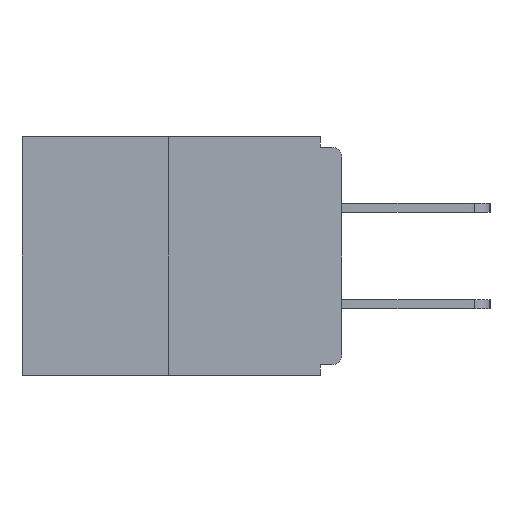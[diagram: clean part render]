
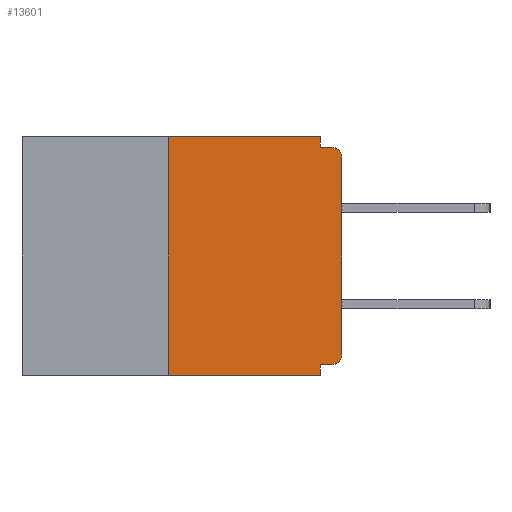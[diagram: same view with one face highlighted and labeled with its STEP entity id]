
A CAD part, left-side view. The second image highlights one B-rep face of the part: STEP entity #13601.
In plain terms, the highlighted planar face has unit normal (-1, 0, 0).
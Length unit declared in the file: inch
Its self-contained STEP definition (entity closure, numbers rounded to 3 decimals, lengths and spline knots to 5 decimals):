
#199 = ORIENTED_EDGE ( 'NONE', *, *, #3254, .F. ) ;
#528 = CARTESIAN_POINT ( 'NONE',  ( 0., 0.015, -0.328 ) ) ;
#533 = VERTEX_POINT ( 'NONE', #11668 ) ;
#868 = LINE ( 'NONE', #8598, #15008 ) ;
#1025 = CARTESIAN_POINT ( 'NONE',  ( 0., 0., 0. ) ) ;
#1148 = DIRECTION ( 'NONE',  ( 0., -1., 0. ) ) ;
#1209 = CARTESIAN_POINT ( 'NONE',  ( 0., 0.25, -0.343 ) ) ;
#1368 = CARTESIAN_POINT ( 'NONE',  ( 0., 0.031, -0.343 ) ) ;
#1601 = LINE ( 'NONE', #5882, #2080 ) ;
#2080 = VECTOR ( 'NONE', #10331, 39.37008 ) ;
#2097 = EDGE_CURVE ( 'NONE', #9857, #6369, #3973, .T. ) ;
#3080 = VERTEX_POINT ( 'NONE', #7480 ) ;
#3254 = EDGE_CURVE ( 'NONE', #533, #16850, #6962, .T. ) ;
#3834 = VECTOR ( 'NONE', #8812, 39.37008 ) ;
#3973 = LINE ( 'NONE', #11247, #7440 ) ;
#4348 = FACE_OUTER_BOUND ( 'NONE', #14300, .T. ) ;
#4618 = VERTEX_POINT ( 'NONE', #8469 ) ;
#5040 = CARTESIAN_POINT ( 'NONE',  ( 0., 0.031, -0.343 ) ) ;
#5282 = EDGE_CURVE ( 'NONE', #18631, #4618, #1601, .T. ) ;
#5661 = EDGE_CURVE ( 'NONE', #16668, #10825, #8485, .T. ) ;
#5882 = CARTESIAN_POINT ( 'NONE',  ( 0., 0.25, 0. ) ) ;
#6029 = PLANE ( 'NONE',  #18758 ) ;
#6369 = VERTEX_POINT ( 'NONE', #8794 ) ;
#6962 = LINE ( 'NONE', #5040, #17421 ) ;
#7039 = ORIENTED_EDGE ( 'NONE', *, *, #16143, .F. ) ;
#7192 = LINE ( 'NONE', #1025, #10149 ) ;
#7356 = ORIENTED_EDGE ( 'NONE', *, *, #10472, .T. ) ;
#7440 = VECTOR ( 'NONE', #1148, 39.37008 ) ;
#7480 = CARTESIAN_POINT ( 'NONE',  ( 0., 0.031, 0. ) ) ;
#7572 = CARTESIAN_POINT ( 'NONE',  ( 0., 0.031, 0. ) ) ;
#7769 = CIRCLE ( 'NONE', #17304, 0.015 ) ;
#8296 = VERTEX_POINT ( 'NONE', #9148 ) ;
#8469 = CARTESIAN_POINT ( 'NONE',  ( 0., 0.25, 0. ) ) ;
#8485 = CIRCLE ( 'NONE', #10786, 0.015 ) ;
#8598 = CARTESIAN_POINT ( 'NONE',  ( 0., 0., -0.328 ) ) ;
#8685 = DIRECTION ( 'NONE',  ( 0., 0., -1. ) ) ;
#8713 = DIRECTION ( 'NONE',  ( 0., 0., -1. ) ) ;
#8794 = CARTESIAN_POINT ( 'NONE',  ( 0., 0.015, -0.015 ) ) ;
#8811 = CARTESIAN_POINT ( 'NONE',  ( 0., 0., -0.313 ) ) ;
#8812 = DIRECTION ( 'NONE',  ( 0., -1., 0. ) ) ;
#9049 = VECTOR ( 'NONE', #15526, 39.37008 ) ;
#9148 = CARTESIAN_POINT ( 'NONE',  ( 0., 0., -0.03 ) ) ;
#9426 = ORIENTED_EDGE ( 'NONE', *, *, #14720, .T. ) ;
#9807 = DIRECTION ( 'NONE',  ( 0., 0., 1. ) ) ;
#9857 = VERTEX_POINT ( 'NONE', #10898 ) ;
#10149 = VECTOR ( 'NONE', #9807, 39.37008 ) ;
#10330 = ORIENTED_EDGE ( 'NONE', *, *, #14773, .F. ) ;
#10331 = DIRECTION ( 'NONE',  ( 0., 0., 1. ) ) ;
#10350 = DIRECTION ( 'NONE',  ( 1., 0., 0. ) ) ;
#10472 = EDGE_CURVE ( 'NONE', #18631, #16850, #12883, .T. ) ;
#10786 = AXIS2_PLACEMENT_3D ( 'NONE', #16102, #13264, #17585 ) ;
#10791 = ORIENTED_EDGE ( 'NONE', *, *, #5282, .F. ) ;
#10825 = VERTEX_POINT ( 'NONE', #8811 ) ;
#10898 = CARTESIAN_POINT ( 'NONE',  ( 0., 0.031, -0.015 ) ) ;
#11247 = CARTESIAN_POINT ( 'NONE',  ( 0., 0., -0.015 ) ) ;
#11385 = LINE ( 'NONE', #17426, #3834 ) ;
#11668 = CARTESIAN_POINT ( 'NONE',  ( 0., 0.031, -0.328 ) ) ;
#11681 = EDGE_CURVE ( 'NONE', #10825, #8296, #7192, .T. ) ;
#11688 = VECTOR ( 'NONE', #16380, 39.37008 ) ;
#12364 = LINE ( 'NONE', #7572, #11688 ) ;
#12883 = LINE ( 'NONE', #18602, #9049 ) ;
#12914 = CARTESIAN_POINT ( 'NONE',  ( 0., 0.015, -0.03 ) ) ;
#12968 = EDGE_CURVE ( 'NONE', #3080, #9857, #12364, .T. ) ;
#13038 = ORIENTED_EDGE ( 'NONE', *, *, #2097, .F. ) ;
#13080 = ORIENTED_EDGE ( 'NONE', *, *, #5661, .T. ) ;
#13199 = ORIENTED_EDGE ( 'NONE', *, *, #11681, .T. ) ;
#13264 = DIRECTION ( 'NONE',  ( -1., 0., 0. ) ) ;
#13601 = ADVANCED_FACE ( 'NONE', ( #4348 ), #6029, .F. ) ;
#14300 = EDGE_LOOP ( 'NONE', ( #10330, #10791, #7356, #199, #7039, #13080, #13199, #9426, #13038, #16296 ) ) ;
#14307 = DIRECTION ( 'NONE',  ( -1., 0., 0. ) ) ;
#14720 = EDGE_CURVE ( 'NONE', #8296, #6369, #7769, .T. ) ;
#14773 = EDGE_CURVE ( 'NONE', #4618, #3080, #11385, .T. ) ;
#15008 = VECTOR ( 'NONE', #18865, 39.37008 ) ;
#15526 = DIRECTION ( 'NONE',  ( 0., -1., 0. ) ) ;
#16102 = CARTESIAN_POINT ( 'NONE',  ( 0., 0.015, -0.313 ) ) ;
#16143 = EDGE_CURVE ( 'NONE', #16668, #533, #868, .T. ) ;
#16296 = ORIENTED_EDGE ( 'NONE', *, *, #12968, .F. ) ;
#16328 = DIRECTION ( 'NONE',  ( 0., 0., -1. ) ) ;
#16380 = DIRECTION ( 'NONE',  ( 0., 0., -1. ) ) ;
#16668 = VERTEX_POINT ( 'NONE', #528 ) ;
#16850 = VERTEX_POINT ( 'NONE', #1368 ) ;
#17304 = AXIS2_PLACEMENT_3D ( 'NONE', #12914, #14307, #8685 ) ;
#17421 = VECTOR ( 'NONE', #16328, 39.37008 ) ;
#17426 = CARTESIAN_POINT ( 'NONE',  ( 0., 0.46, 0. ) ) ;
#17585 = DIRECTION ( 'NONE',  ( 0., 0., -1. ) ) ;
#17597 = CARTESIAN_POINT ( 'NONE',  ( 0., 0.46, 0. ) ) ;
#18602 = CARTESIAN_POINT ( 'NONE',  ( 0., 0.46, -0.343 ) ) ;
#18631 = VERTEX_POINT ( 'NONE', #1209 ) ;
#18758 = AXIS2_PLACEMENT_3D ( 'NONE', #17597, #10350, #8713 ) ;
#18865 = DIRECTION ( 'NONE',  ( 0., 1., 0. ) ) ;
